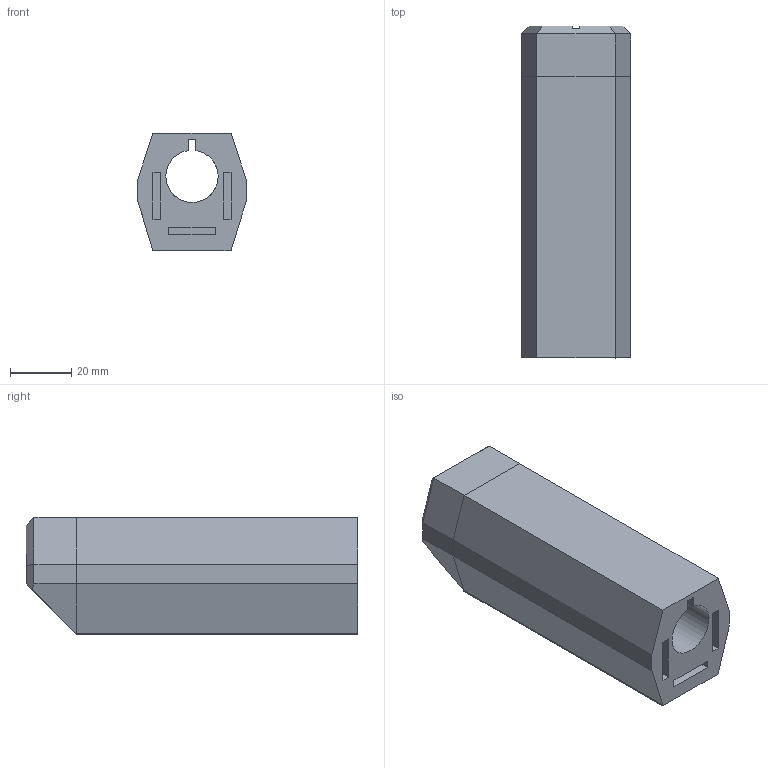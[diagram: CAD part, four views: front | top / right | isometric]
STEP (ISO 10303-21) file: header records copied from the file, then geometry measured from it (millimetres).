
FILE_DESCRIPTION(/* description */ (''),/* implementation_level */ '2;1');
FILE_NAME(/* name */ 'c7f97ce9-3479-4d9c-bf3b-c72360efb5c8.stp',/* time_stamp */ '2019-11-26T06:32:33+00:00',/* author */ (''),/* organization */ (''),/* preprocessor_version */ 'ST-DEVELOPER v18',/* originating_system */ 'Autodesk Translation Framework v8.12.0.6',/* authorisation */ '');
FILE_SCHEMA (('AUTOMOTIVE_DESIGN { 1 0 10303 214 3 1 1 }'));
Length unit declared in the file: inch
Products named in the file (1): HRR Foreend Cap
Bounding box: 35.56 x 107.95 x 38.1 mm (x, y, z)
Volume: 98322.9 mm3; surface area: 27154.1 mm2
Topology: 4 solids, 4 shells, 82 faces, 215 edges, 142 vertices
Faces by surface type: plane 80, cylinder 2
Entity records: 2525 total; most frequent: CARTESIAN_POINT 440, ORIENTED_EDGE 430, DIRECTION 387, EDGE_CURVE 215, LINE 209, VECTOR 209, VERTEX_POINT 142, EDGE_LOOP 93
